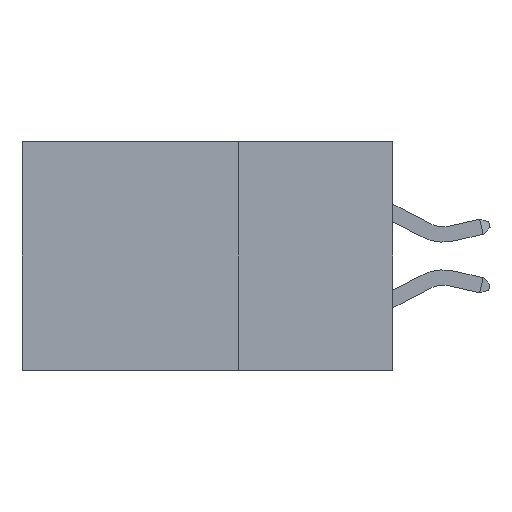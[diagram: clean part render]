
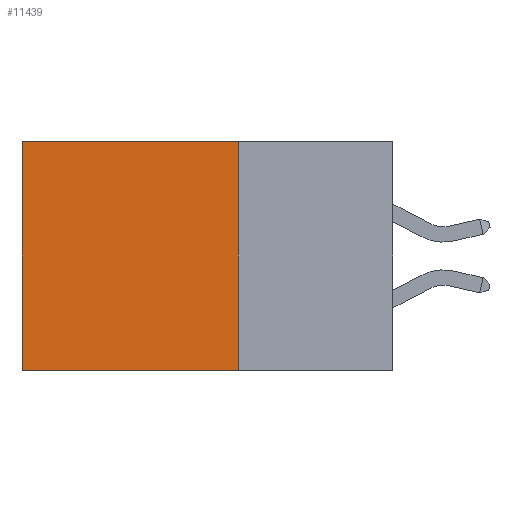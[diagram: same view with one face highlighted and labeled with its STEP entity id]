
A CAD part, left-side view. The second image highlights one B-rep face of the part: STEP entity #11439.
In plain terms, the highlighted planar face has unit normal (-1, 0, 0).
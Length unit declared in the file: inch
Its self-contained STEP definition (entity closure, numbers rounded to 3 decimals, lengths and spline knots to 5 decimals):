
#339 = EDGE_CURVE ( 'NONE', #4515, #14441, #11638, .T. ) ;
#430 = DIRECTION ( 'NONE',  ( 0., 0., -1. ) ) ;
#1519 = EDGE_CURVE ( 'NONE', #10447, #4515, #6360, .T. ) ;
#1639 = EDGE_LOOP ( 'NONE', ( #2140, #5592, #8620, #6863 ) ) ;
#1925 = DIRECTION ( 'NONE',  ( 1., 0., 0. ) ) ;
#2082 = EDGE_CURVE ( 'NONE', #10447, #11796, #2489, .T. ) ;
#2140 = ORIENTED_EDGE ( 'NONE', *, *, #13223, .T. ) ;
#2489 = LINE ( 'NONE', #4488, #15251 ) ;
#2678 = VECTOR ( 'NONE', #4769, 39.37008 ) ;
#2735 = CARTESIAN_POINT ( 'NONE',  ( 0.2875, 0.25, 0. ) ) ;
#4383 = CARTESIAN_POINT ( 'NONE',  ( 0.2875, 0.6, -0.37 ) ) ;
#4488 = CARTESIAN_POINT ( 'NONE',  ( 0.2875, 0.25, 0. ) ) ;
#4515 = VERTEX_POINT ( 'NONE', #12975 ) ;
#4769 = DIRECTION ( 'NONE',  ( 0., 0., -1. ) ) ;
#5052 = VECTOR ( 'NONE', #6597, 39.37008 ) ;
#5592 = ORIENTED_EDGE ( 'NONE', *, *, #339, .F. ) ;
#6360 = LINE ( 'NONE', #10945, #2678 ) ;
#6597 = DIRECTION ( 'NONE',  ( 0., 1., 0. ) ) ;
#6863 = ORIENTED_EDGE ( 'NONE', *, *, #2082, .T. ) ;
#7383 = VECTOR ( 'NONE', #430, 39.37008 ) ;
#8597 = FACE_OUTER_BOUND ( 'NONE', #1639, .T. ) ;
#8620 = ORIENTED_EDGE ( 'NONE', *, *, #1519, .F. ) ;
#9393 = PLANE ( 'NONE',  #12820 ) ;
#9468 = DIRECTION ( 'NONE',  ( 0., 1., 0. ) ) ;
#10182 = CARTESIAN_POINT ( 'NONE',  ( 0.2875, 0.6, 0. ) ) ;
#10447 = VERTEX_POINT ( 'NONE', #2735 ) ;
#10540 = CARTESIAN_POINT ( 'NONE',  ( 0.2875, 0.6, 0. ) ) ;
#10649 = DIRECTION ( 'NONE',  ( 0., 0., -1. ) ) ;
#10793 = CARTESIAN_POINT ( 'NONE',  ( 0.2875, 0.25, -0.37 ) ) ;
#10945 = CARTESIAN_POINT ( 'NONE',  ( 0.2875, 0.25, 0. ) ) ;
#11439 = ADVANCED_FACE ( 'NONE', ( #8597 ), #9393, .F. ) ;
#11638 = LINE ( 'NONE', #10793, #5052 ) ;
#11796 = VERTEX_POINT ( 'NONE', #10182 ) ;
#12820 = AXIS2_PLACEMENT_3D ( 'NONE', #15505, #1925, #10649 ) ;
#12975 = CARTESIAN_POINT ( 'NONE',  ( 0.2875, 0.25, -0.37 ) ) ;
#13223 = EDGE_CURVE ( 'NONE', #11796, #14441, #13942, .T. ) ;
#13942 = LINE ( 'NONE', #10540, #7383 ) ;
#14441 = VERTEX_POINT ( 'NONE', #4383 ) ;
#15251 = VECTOR ( 'NONE', #9468, 39.37008 ) ;
#15505 = CARTESIAN_POINT ( 'NONE',  ( 0.2875, 0.25, 0. ) ) ;
